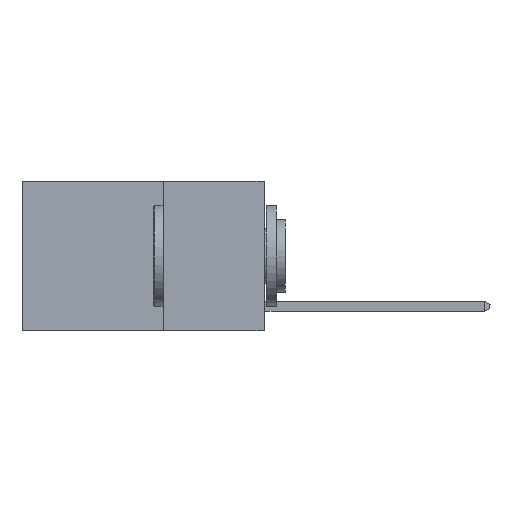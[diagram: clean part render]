
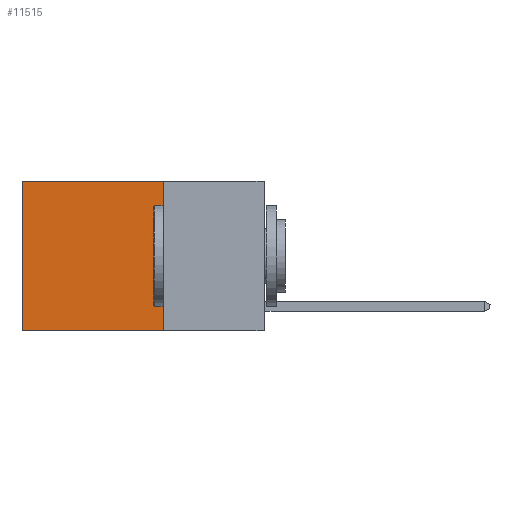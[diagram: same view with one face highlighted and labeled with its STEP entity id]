
A CAD part, left-side view. The second image highlights one B-rep face of the part: STEP entity #11515.
In plain terms, the highlighted planar face has unit normal (-1, 0, 0).
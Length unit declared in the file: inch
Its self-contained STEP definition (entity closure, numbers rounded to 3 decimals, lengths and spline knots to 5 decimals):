
#356 = VERTEX_POINT ( 'NONE', #9658 ) ;
#929 = VECTOR ( 'NONE', #5542, 39.37008 ) ;
#1356 = ORIENTED_EDGE ( 'NONE', *, *, #10128, .F. ) ;
#1415 = ORIENTED_EDGE ( 'NONE', *, *, #2902, .T. ) ;
#2080 = AXIS2_PLACEMENT_3D ( 'NONE', #11692, #12683, #6375 ) ;
#2248 = VERTEX_POINT ( 'NONE', #7868 ) ;
#2902 = EDGE_CURVE ( 'NONE', #356, #8314, #3490, .T. ) ;
#3490 = LINE ( 'NONE', #11914, #929 ) ;
#4303 = DIRECTION ( 'NONE',  ( 0., 1., 0. ) ) ;
#4380 = DIRECTION ( 'NONE',  ( 0., 0., -1. ) ) ;
#4629 = VECTOR ( 'NONE', #6772, 39.37008 ) ;
#5310 = PLANE ( 'NONE',  #2080 ) ;
#5542 = DIRECTION ( 'NONE',  ( 0., 1., 0. ) ) ;
#5685 = CARTESIAN_POINT ( 'NONE',  ( 0.2625, 0.25, 0. ) ) ;
#5804 = VECTOR ( 'NONE', #4303, 39.37008 ) ;
#5806 = VERTEX_POINT ( 'NONE', #12331 ) ;
#6375 = DIRECTION ( 'NONE',  ( 0., 0., -1. ) ) ;
#6427 = FACE_OUTER_BOUND ( 'NONE', #9531, .T. ) ;
#6772 = DIRECTION ( 'NONE',  ( 0., 0., -1. ) ) ;
#7868 = CARTESIAN_POINT ( 'NONE',  ( 0.2625, 0.25, -0.37 ) ) ;
#8117 = EDGE_CURVE ( 'NONE', #356, #2248, #10339, .T. ) ;
#8118 = LINE ( 'NONE', #11797, #10570 ) ;
#8314 = VERTEX_POINT ( 'NONE', #12330 ) ;
#8915 = EDGE_CURVE ( 'NONE', #8314, #5806, #8118, .T. ) ;
#9531 = EDGE_LOOP ( 'NONE', ( #10697, #1356, #11204, #1415 ) ) ;
#9658 = CARTESIAN_POINT ( 'NONE',  ( 0.2625, 0.25, 0. ) ) ;
#9689 = CARTESIAN_POINT ( 'NONE',  ( 0.2625, 0.25, -0.37 ) ) ;
#10128 = EDGE_CURVE ( 'NONE', #2248, #5806, #11499, .T. ) ;
#10339 = LINE ( 'NONE', #5685, #4629 ) ;
#10570 = VECTOR ( 'NONE', #4380, 39.37008 ) ;
#10697 = ORIENTED_EDGE ( 'NONE', *, *, #8915, .T. ) ;
#11204 = ORIENTED_EDGE ( 'NONE', *, *, #8117, .F. ) ;
#11499 = LINE ( 'NONE', #9689, #5804 ) ;
#11515 = ADVANCED_FACE ( 'NONE', ( #6427 ), #5310, .F. ) ;
#11692 = CARTESIAN_POINT ( 'NONE',  ( 0.2625, 0.25, 0. ) ) ;
#11797 = CARTESIAN_POINT ( 'NONE',  ( 0.2625, 0.6, 0. ) ) ;
#11914 = CARTESIAN_POINT ( 'NONE',  ( 0.2625, 0.25, 0. ) ) ;
#12330 = CARTESIAN_POINT ( 'NONE',  ( 0.2625, 0.6, 0. ) ) ;
#12331 = CARTESIAN_POINT ( 'NONE',  ( 0.2625, 0.6, -0.37 ) ) ;
#12683 = DIRECTION ( 'NONE',  ( 1., 0., 0. ) ) ;
